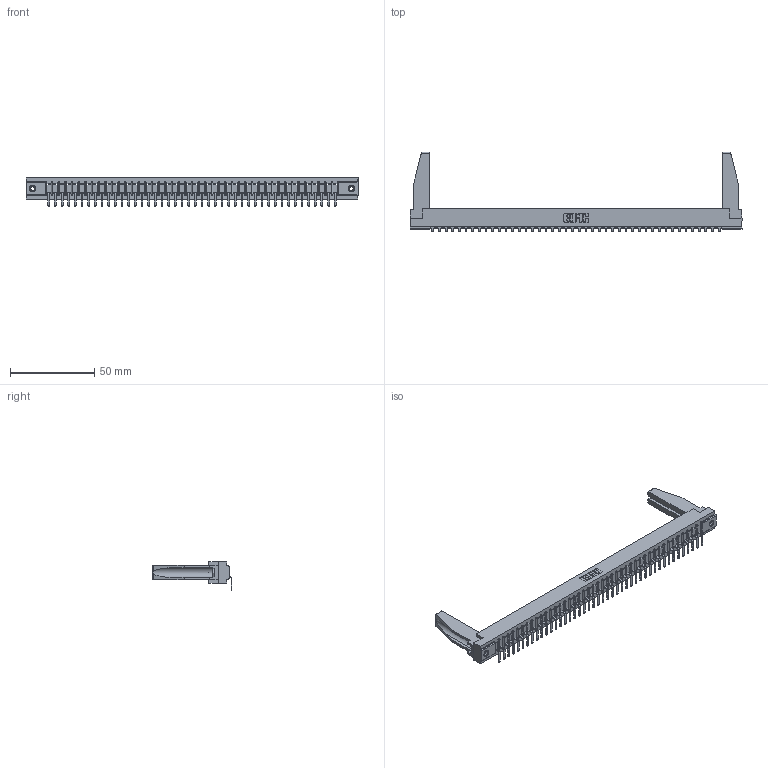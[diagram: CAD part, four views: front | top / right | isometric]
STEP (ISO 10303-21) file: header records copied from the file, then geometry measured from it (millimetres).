
FILE_DESCRIPTION (( 'STEP AP203' ), '1' );
FILE_NAME ('357-044-559-178.STEP', '2022-07-12T19:21:06', ( '' ), ( '' ), 'SwSTEP 2.0', 'SolidWorks 2020', '' );
FILE_SCHEMA (( 'CONFIG_CONTROL_DESIGN' ));
Length unit declared in the file: inch
Products named in the file (5): 307-290-001_558 559 - 1 (Single); 357-044-559-178; 307 Part_.156 Dia Mounting Holes; 345-250-001_345-250-001-102; 307-220-078
Assembly tree (49 placements, depth 2):
  357-044-559-178
    307 Part_.156 Dia Mounting Holes
    307-290-001_558 559 - 1 (Single)  x44
    307-220-078  x2
    345-250-001_345-250-001-102  x2
Bounding box: 197.36 x 47.41 x 16.8 mm (x, y, z)
Volume: 24517 mm3; surface area: 25702.5 mm2
Topology: 49 solids, 49 shells, 2933 faces, 8309 edges, 5350 vertices
Faces by surface type: plane 1870, cylinder 957, sphere 90, cone 12, torus 4
Entity records: 40017 total; most frequent: CARTESIAN_POINT 6742, ORIENTED_EDGE 6684, DIRECTION 6512, EDGE_CURVE 3342, LINE 2568, VECTOR 2568, VERTEX_POINT 2160, AXIS2_PLACEMENT_3D 1972
